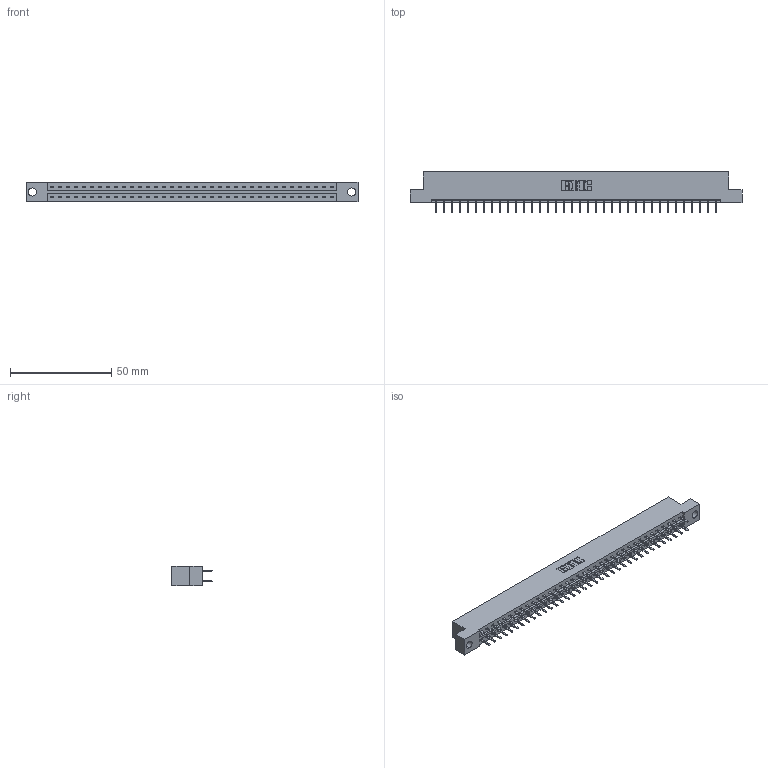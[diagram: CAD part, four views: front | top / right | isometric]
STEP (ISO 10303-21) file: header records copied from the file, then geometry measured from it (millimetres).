
FILE_DESCRIPTION (( 'STEP AP203' ), '1' );
FILE_NAME ('833-072-520-204.STEP', '2020-06-05T13:39:16', ( '' ), ( '' ), 'SwSTEP 2.0', 'SolidWorks 2020', '' );
FILE_SCHEMA (( 'CONFIG_CONTROL_DESIGN' ));
Length unit declared in the file: inch
Products named in the file (3): 833-072-520-204; 345-292-001_345-293-120; 833 Part_Flush - .156 Dia - TH
Assembly tree (73 placements, depth 2):
  833-072-520-204
    833 Part_Flush - .156 Dia - TH
    345-292-001_345-293-120  x72
Bounding box: 164.19 x 20.02 x 9.4 mm (x, y, z)
Volume: 16586.8 mm3; surface area: 19260.8 mm2
Topology: 73 solids, 73 shells, 4146 faces, 12047 edges, 7838 vertices
Faces by surface type: plane 2806, cylinder 1340
Entity records: 24053 total; most frequent: CARTESIAN_POINT 4006, ORIENTED_EDGE 3930, DIRECTION 3421, EDGE_CURVE 1965, VECTOR 1833, LINE 1833, VERTEX_POINT 1306, AXIS2_PLACEMENT_3D 794
